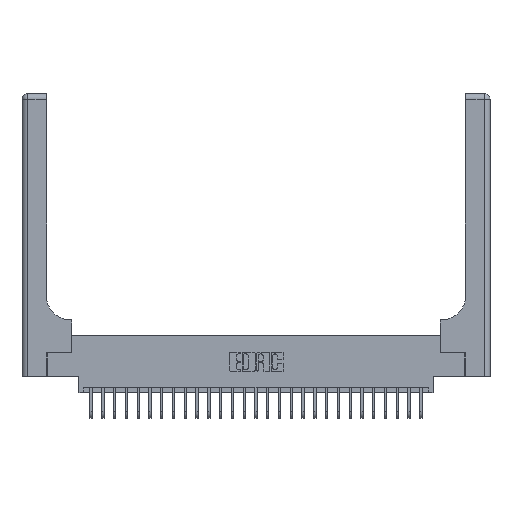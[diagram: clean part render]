
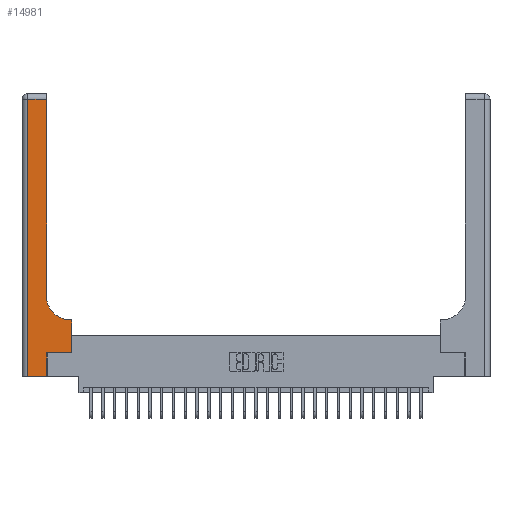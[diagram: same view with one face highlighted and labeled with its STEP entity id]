
A CAD part, top view. The second image highlights one B-rep face of the part: STEP entity #14981.
In plain terms, the highlighted planar face has unit normal (0, 0, 1).
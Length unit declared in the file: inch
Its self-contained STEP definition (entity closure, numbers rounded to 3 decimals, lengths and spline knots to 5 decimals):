
#370 = DIRECTION ( 'NONE',  ( -1., 0., 0. ) ) ;
#895 = EDGE_CURVE ( 'NONE', #27391, #8542, #20639, .T. ) ;
#920 = CARTESIAN_POINT ( 'NONE',  ( 0., 0., 0.37 ) ) ;
#1048 = CARTESIAN_POINT ( 'NONE',  ( 0.26, 0.6, 0.37 ) ) ;
#1126 = VERTEX_POINT ( 'NONE', #4173 ) ;
#1556 = VERTEX_POINT ( 'NONE', #6300 ) ;
#2307 = LINE ( 'NONE', #24032, #7428 ) ;
#2687 = LINE ( 'NONE', #20281, #3735 ) ;
#3386 = DIRECTION ( 'NONE',  ( 0., 1., 0. ) ) ;
#3431 = CARTESIAN_POINT ( 'NONE',  ( 0.265, 0.25, 0.37 ) ) ;
#3646 = CARTESIAN_POINT ( 'NONE',  ( 0.51, 0.6, 0.37 ) ) ;
#3708 = LINE ( 'NONE', #3431, #11801 ) ;
#3735 = VECTOR ( 'NONE', #13425, 39.37008 ) ;
#3841 = CARTESIAN_POINT ( 'NONE',  ( 0.26, 0.85, 0.37 ) ) ;
#4138 = VERTEX_POINT ( 'NONE', #9779 ) ;
#4173 = CARTESIAN_POINT ( 'NONE',  ( 0.528, 0.25, 0.37 ) ) ;
#5504 = CARTESIAN_POINT ( 'NONE',  ( 0.06, 3., 0.37 ) ) ;
#6300 = CARTESIAN_POINT ( 'NONE',  ( 0.06, 2.94, 0.37 ) ) ;
#6770 = EDGE_CURVE ( 'NONE', #1556, #4138, #13678, .T. ) ;
#7428 = VECTOR ( 'NONE', #19628, 39.37008 ) ;
#7491 = VECTOR ( 'NONE', #13527, 39.37008 ) ;
#7552 = LINE ( 'NONE', #22821, #8648 ) ;
#7867 = DIRECTION ( 'NONE',  ( 1., 0., 0. ) ) ;
#8542 = VERTEX_POINT ( 'NONE', #3646 ) ;
#8648 = VECTOR ( 'NONE', #3386, 39.37008 ) ;
#8751 = AXIS2_PLACEMENT_3D ( 'NONE', #16984, #25687, #14859 ) ;
#9140 = ORIENTED_EDGE ( 'NONE', *, *, #25732, .T. ) ;
#9378 = FACE_OUTER_BOUND ( 'NONE', #19266, .T. ) ;
#9522 = EDGE_CURVE ( 'NONE', #12332, #1126, #3708, .T. ) ;
#9779 = CARTESIAN_POINT ( 'NONE',  ( 0.06, 0., 0.37 ) ) ;
#9785 = DIRECTION ( 'NONE',  ( -1., 0., 0. ) ) ;
#10009 = VERTEX_POINT ( 'NONE', #10406 ) ;
#10406 = CARTESIAN_POINT ( 'NONE',  ( 0.265, 0., 0.37 ) ) ;
#11801 = VECTOR ( 'NONE', #7867, 39.37008 ) ;
#11967 = AXIS2_PLACEMENT_3D ( 'NONE', #19813, #26504, #370 ) ;
#12332 = VERTEX_POINT ( 'NONE', #19769 ) ;
#12363 = ORIENTED_EDGE ( 'NONE', *, *, #6770, .T. ) ;
#13425 = DIRECTION ( 'NONE',  ( 0., 1., 0. ) ) ;
#13527 = DIRECTION ( 'NONE',  ( 1., 0., 0. ) ) ;
#13673 = LINE ( 'NONE', #920, #7491 ) ;
#13678 = LINE ( 'NONE', #5504, #14414 ) ;
#13785 = ORIENTED_EDGE ( 'NONE', *, *, #15467, .T. ) ;
#14414 = VECTOR ( 'NONE', #18233, 39.37008 ) ;
#14466 = EDGE_CURVE ( 'NONE', #8542, #27204, #15600, .T. ) ;
#14859 = DIRECTION ( 'NONE',  ( 1., 0., 0. ) ) ;
#14981 = ADVANCED_FACE ( 'NONE', ( #9378 ), #19968, .F. ) ;
#15467 = EDGE_CURVE ( 'NONE', #27204, #18267, #27158, .T. ) ;
#15600 = CIRCLE ( 'NONE', #8751, 0.25 ) ;
#15786 = EDGE_CURVE ( 'NONE', #10009, #12332, #2687, .T. ) ;
#15897 = ORIENTED_EDGE ( 'NONE', *, *, #15786, .T. ) ;
#16315 = CARTESIAN_POINT ( 'NONE',  ( 0.26, 3., 0.37 ) ) ;
#16323 = EDGE_CURVE ( 'NONE', #18267, #1556, #2307, .T. ) ;
#16984 = CARTESIAN_POINT ( 'NONE',  ( 0.51, 0.85, 0.37 ) ) ;
#17265 = ORIENTED_EDGE ( 'NONE', *, *, #17307, .T. ) ;
#17307 = EDGE_CURVE ( 'NONE', #4138, #10009, #13673, .T. ) ;
#17456 = VECTOR ( 'NONE', #26578, 39.37008 ) ;
#18233 = DIRECTION ( 'NONE',  ( 0., -1., 0. ) ) ;
#18267 = VERTEX_POINT ( 'NONE', #19882 ) ;
#19133 = ORIENTED_EDGE ( 'NONE', *, *, #9522, .T. ) ;
#19266 = EDGE_LOOP ( 'NONE', ( #13785, #20353, #12363, #17265, #15897, #19133, #9140, #21736, #26629 ) ) ;
#19628 = DIRECTION ( 'NONE',  ( -1., 0., 0. ) ) ;
#19715 = CARTESIAN_POINT ( 'NONE',  ( 0.528, 0.6, 0.37 ) ) ;
#19769 = CARTESIAN_POINT ( 'NONE',  ( 0.265, 0.25, 0.37 ) ) ;
#19813 = CARTESIAN_POINT ( 'NONE',  ( 0., 3., 0.37 ) ) ;
#19882 = CARTESIAN_POINT ( 'NONE',  ( 0.26, 2.94, 0.37 ) ) ;
#19968 = PLANE ( 'NONE',  #11967 ) ;
#20281 = CARTESIAN_POINT ( 'NONE',  ( 0.265, 0., 0.37 ) ) ;
#20353 = ORIENTED_EDGE ( 'NONE', *, *, #16323, .T. ) ;
#20639 = LINE ( 'NONE', #1048, #25627 ) ;
#21736 = ORIENTED_EDGE ( 'NONE', *, *, #895, .T. ) ;
#22821 = CARTESIAN_POINT ( 'NONE',  ( 0.528, 0.25, 0.37 ) ) ;
#24032 = CARTESIAN_POINT ( 'NONE',  ( 0., 2.94, 0.37 ) ) ;
#25627 = VECTOR ( 'NONE', #9785, 39.37008 ) ;
#25687 = DIRECTION ( 'NONE',  ( 0., 0., -1. ) ) ;
#25732 = EDGE_CURVE ( 'NONE', #1126, #27391, #7552, .T. ) ;
#26504 = DIRECTION ( 'NONE',  ( 0., 0., -1. ) ) ;
#26578 = DIRECTION ( 'NONE',  ( 0., 1., 0. ) ) ;
#26629 = ORIENTED_EDGE ( 'NONE', *, *, #14466, .T. ) ;
#27158 = LINE ( 'NONE', #16315, #17456 ) ;
#27204 = VERTEX_POINT ( 'NONE', #3841 ) ;
#27391 = VERTEX_POINT ( 'NONE', #19715 ) ;
